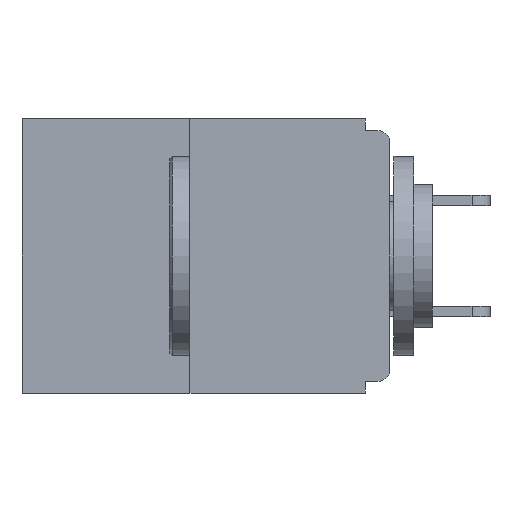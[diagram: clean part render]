
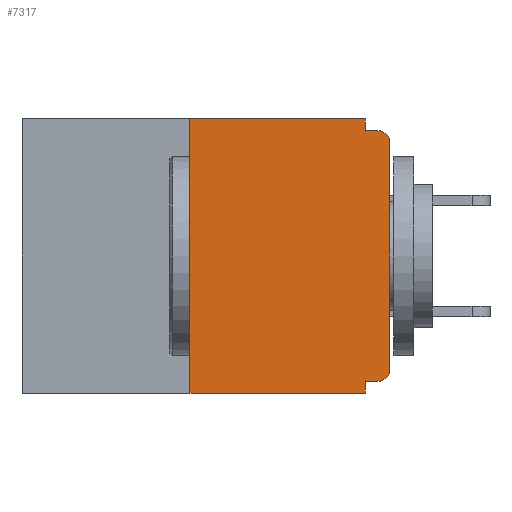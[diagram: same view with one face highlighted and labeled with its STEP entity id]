
A CAD part, left-side view. The second image highlights one B-rep face of the part: STEP entity #7317.
In plain terms, the highlighted planar face has unit normal (-1, 0, 0).
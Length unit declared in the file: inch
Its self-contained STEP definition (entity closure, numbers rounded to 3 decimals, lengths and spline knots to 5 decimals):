
#56 = VERTEX_POINT ( 'NONE', #20064 ) ;
#135 = CARTESIAN_POINT ( 'NONE',  ( 0., 0.46, 0. ) ) ;
#603 = VERTEX_POINT ( 'NONE', #3743 ) ;
#953 = VERTEX_POINT ( 'NONE', #23826 ) ;
#1311 = EDGE_CURVE ( 'NONE', #603, #6242, #7363, .T. ) ;
#1393 = VERTEX_POINT ( 'NONE', #7843 ) ;
#1454 = DIRECTION ( 'NONE',  ( 0., 0., 1. ) ) ;
#1520 = AXIS2_PLACEMENT_3D ( 'NONE', #20610, #2465, #18677 ) ;
#1539 = EDGE_CURVE ( 'NONE', #603, #12421, #14633, .T. ) ;
#1657 = EDGE_CURVE ( 'NONE', #1393, #6453, #16202, .T. ) ;
#1812 = CIRCLE ( 'NONE', #4588, 0.015 ) ;
#2465 = DIRECTION ( 'NONE',  ( 1., 0., 0. ) ) ;
#2572 = VECTOR ( 'NONE', #3732, 39.37008 ) ;
#3039 = ORIENTED_EDGE ( 'NONE', *, *, #17022, .F. ) ;
#3267 = ORIENTED_EDGE ( 'NONE', *, *, #7796, .T. ) ;
#3433 = EDGE_CURVE ( 'NONE', #15992, #14738, #13309, .T. ) ;
#3732 = DIRECTION ( 'NONE',  ( 0., -1., 0. ) ) ;
#3743 = CARTESIAN_POINT ( 'NONE',  ( 0., 0.25, -0.343 ) ) ;
#4173 = DIRECTION ( 'NONE',  ( 0., -1., 0. ) ) ;
#4391 = PLANE ( 'NONE',  #1520 ) ;
#4572 = DIRECTION ( 'NONE',  ( 0., 0., -1. ) ) ;
#4588 = AXIS2_PLACEMENT_3D ( 'NONE', #19328, #7246, #21366 ) ;
#5369 = AXIS2_PLACEMENT_3D ( 'NONE', #13717, #23684, #15650 ) ;
#5633 = CARTESIAN_POINT ( 'NONE',  ( 0., 0., -0.313 ) ) ;
#5696 = LINE ( 'NONE', #12033, #12049 ) ;
#5742 = LINE ( 'NONE', #8872, #23164 ) ;
#6038 = EDGE_CURVE ( 'NONE', #953, #6242, #13946, .T. ) ;
#6242 = VERTEX_POINT ( 'NONE', #15096 ) ;
#6453 = VERTEX_POINT ( 'NONE', #5633 ) ;
#7242 = CARTESIAN_POINT ( 'NONE',  ( 0., 0.031, 0. ) ) ;
#7246 = DIRECTION ( 'NONE',  ( -1., 0., 0. ) ) ;
#7317 = ADVANCED_FACE ( 'NONE', ( #18948 ), #4391, .F. ) ;
#7363 = LINE ( 'NONE', #17923, #2572 ) ;
#7796 = EDGE_CURVE ( 'NONE', #56, #8574, #1812, .T. ) ;
#7843 = CARTESIAN_POINT ( 'NONE',  ( 0., 0.015, -0.328 ) ) ;
#8574 = VERTEX_POINT ( 'NONE', #14133 ) ;
#8836 = ORIENTED_EDGE ( 'NONE', *, *, #13926, .F. ) ;
#8872 = CARTESIAN_POINT ( 'NONE',  ( 0., 0., -0.015 ) ) ;
#10546 = DIRECTION ( 'NONE',  ( 0., 0., 1. ) ) ;
#10812 = EDGE_CURVE ( 'NONE', #14738, #8574, #5742, .T. ) ;
#10925 = DIRECTION ( 'NONE',  ( 0., 1., 0. ) ) ;
#10941 = EDGE_LOOP ( 'NONE', ( #3039, #21291, #21136, #13891, #8836, #16414, #16053, #3267, #16393, #13884 ) ) ;
#11740 = CARTESIAN_POINT ( 'NONE',  ( 0., 0.031, 0. ) ) ;
#12033 = CARTESIAN_POINT ( 'NONE',  ( 0., 0., 0. ) ) ;
#12049 = VECTOR ( 'NONE', #1454, 39.37008 ) ;
#12421 = VERTEX_POINT ( 'NONE', #18963 ) ;
#13309 = LINE ( 'NONE', #11740, #24396 ) ;
#13495 = DIRECTION ( 'NONE',  ( 0., -1., 0. ) ) ;
#13534 = CARTESIAN_POINT ( 'NONE',  ( 0., 0.031, -0.015 ) ) ;
#13717 = CARTESIAN_POINT ( 'NONE',  ( 0., 0.015, -0.313 ) ) ;
#13884 = ORIENTED_EDGE ( 'NONE', *, *, #3433, .F. ) ;
#13891 = ORIENTED_EDGE ( 'NONE', *, *, #6038, .F. ) ;
#13926 = EDGE_CURVE ( 'NONE', #1393, #953, #21851, .T. ) ;
#13946 = LINE ( 'NONE', #16723, #23413 ) ;
#14133 = CARTESIAN_POINT ( 'NONE',  ( 0., 0.015, -0.015 ) ) ;
#14633 = LINE ( 'NONE', #16470, #21258 ) ;
#14695 = EDGE_CURVE ( 'NONE', #6453, #56, #5696, .T. ) ;
#14738 = VERTEX_POINT ( 'NONE', #13534 ) ;
#15096 = CARTESIAN_POINT ( 'NONE',  ( 0., 0.031, -0.343 ) ) ;
#15408 = VECTOR ( 'NONE', #4173, 39.37008 ) ;
#15650 = DIRECTION ( 'NONE',  ( 0., 0., -1. ) ) ;
#15992 = VERTEX_POINT ( 'NONE', #7242 ) ;
#16053 = ORIENTED_EDGE ( 'NONE', *, *, #14695, .T. ) ;
#16202 = CIRCLE ( 'NONE', #5369, 0.015 ) ;
#16393 = ORIENTED_EDGE ( 'NONE', *, *, #10812, .F. ) ;
#16414 = ORIENTED_EDGE ( 'NONE', *, *, #1657, .T. ) ;
#16470 = CARTESIAN_POINT ( 'NONE',  ( 0., 0.25, 0. ) ) ;
#16723 = CARTESIAN_POINT ( 'NONE',  ( 0., 0.031, -0.343 ) ) ;
#17022 = EDGE_CURVE ( 'NONE', #12421, #15992, #20768, .T. ) ;
#17923 = CARTESIAN_POINT ( 'NONE',  ( 0., 0.46, -0.343 ) ) ;
#18677 = DIRECTION ( 'NONE',  ( 0., 0., -1. ) ) ;
#18948 = FACE_OUTER_BOUND ( 'NONE', #10941, .T. ) ;
#18963 = CARTESIAN_POINT ( 'NONE',  ( 0., 0.25, 0. ) ) ;
#19328 = CARTESIAN_POINT ( 'NONE',  ( 0., 0.015, -0.03 ) ) ;
#20064 = CARTESIAN_POINT ( 'NONE',  ( 0., 0., -0.03 ) ) ;
#20610 = CARTESIAN_POINT ( 'NONE',  ( 0., 0.46, 0. ) ) ;
#20768 = LINE ( 'NONE', #135, #15408 ) ;
#20973 = CARTESIAN_POINT ( 'NONE',  ( 0., 0., -0.328 ) ) ;
#21136 = ORIENTED_EDGE ( 'NONE', *, *, #1311, .T. ) ;
#21258 = VECTOR ( 'NONE', #10546, 39.37008 ) ;
#21291 = ORIENTED_EDGE ( 'NONE', *, *, #1539, .F. ) ;
#21366 = DIRECTION ( 'NONE',  ( 0., 0., -1. ) ) ;
#21851 = LINE ( 'NONE', #20973, #25345 ) ;
#23164 = VECTOR ( 'NONE', #13495, 39.37008 ) ;
#23413 = VECTOR ( 'NONE', #4572, 39.37008 ) ;
#23684 = DIRECTION ( 'NONE',  ( -1., 0., 0. ) ) ;
#23826 = CARTESIAN_POINT ( 'NONE',  ( 0., 0.031, -0.328 ) ) ;
#24396 = VECTOR ( 'NONE', #25882, 39.37008 ) ;
#25345 = VECTOR ( 'NONE', #10925, 39.37008 ) ;
#25882 = DIRECTION ( 'NONE',  ( 0., 0., -1. ) ) ;
